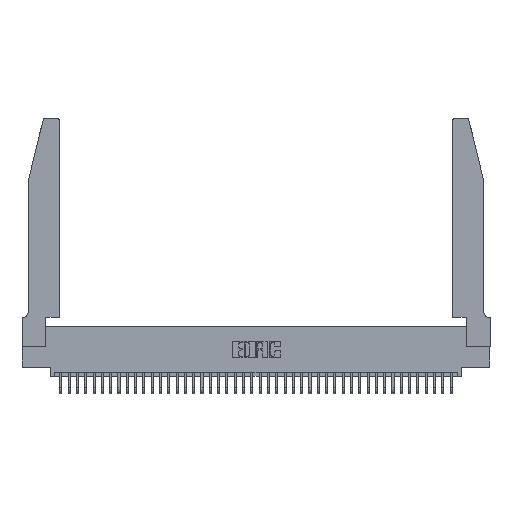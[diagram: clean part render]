
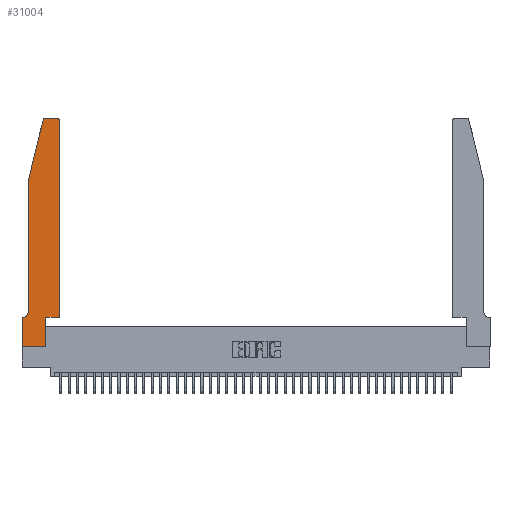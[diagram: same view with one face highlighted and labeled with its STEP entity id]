
A CAD part, top view. The second image highlights one B-rep face of the part: STEP entity #31004.
In plain terms, the highlighted planar face has unit normal (0, 0, 1).
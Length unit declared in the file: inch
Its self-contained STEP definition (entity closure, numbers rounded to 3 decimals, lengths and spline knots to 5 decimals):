
#137 = ORIENTED_EDGE ( 'NONE', *, *, #31049, .T. ) ;
#503 = ORIENTED_EDGE ( 'NONE', *, *, #36519, .T. ) ;
#614 = CARTESIAN_POINT ( 'NONE',  ( 0., 0., 0.37 ) ) ;
#627 = CARTESIAN_POINT ( 'NONE',  ( 0.2865, 0.35, 0.37 ) ) ;
#1128 = VERTEX_POINT ( 'NONE', #8726 ) ;
#1502 = LINE ( 'NONE', #24448, #2562 ) ;
#1801 = VERTEX_POINT ( 'NONE', #23933 ) ;
#1944 = VERTEX_POINT ( 'NONE', #18212 ) ;
#2562 = VECTOR ( 'NONE', #17711, 39.37008 ) ;
#2728 = DIRECTION ( 'NONE',  ( 0., 1., 0. ) ) ;
#3077 = ORIENTED_EDGE ( 'NONE', *, *, #26195, .T. ) ;
#4202 = ORIENTED_EDGE ( 'NONE', *, *, #9732, .T. ) ;
#4625 = VECTOR ( 'NONE', #2728, 39.37008 ) ;
#6936 = LINE ( 'NONE', #20820, #40426 ) ;
#8248 = CARTESIAN_POINT ( 'NONE',  ( 0.0755, 2., 0.37 ) ) ;
#8726 = CARTESIAN_POINT ( 'NONE',  ( 0., 0.35, 0.37 ) ) ;
#8835 = CARTESIAN_POINT ( 'NONE',  ( 0.284, 2.72, 0.37 ) ) ;
#8965 = CIRCLE ( 'NONE', #24056, 0.03 ) ;
#9063 = ORIENTED_EDGE ( 'NONE', *, *, #30540, .T. ) ;
#9194 = VERTEX_POINT ( 'NONE', #18408 ) ;
#9270 = EDGE_CURVE ( 'NONE', #25083, #10269, #41561, .T. ) ;
#9732 = EDGE_CURVE ( 'NONE', #1801, #9194, #25870, .T. ) ;
#10200 = EDGE_CURVE ( 'NONE', #9194, #11248, #6936, .T. ) ;
#10269 = VERTEX_POINT ( 'NONE', #11112 ) ;
#10352 = ORIENTED_EDGE ( 'NONE', *, *, #10200, .T. ) ;
#11086 = EDGE_CURVE ( 'NONE', #10269, #1801, #8965, .T. ) ;
#11112 = CARTESIAN_POINT ( 'NONE',  ( 0.284, 2.75, 0.37 ) ) ;
#11248 = VERTEX_POINT ( 'NONE', #39684 ) ;
#11329 = DIRECTION ( 'NONE',  ( 1., 0., 0. ) ) ;
#11650 = EDGE_CURVE ( 'NONE', #26159, #1128, #13074, .T. ) ;
#11720 = VECTOR ( 'NONE', #37430, 39.37008 ) ;
#12178 = DIRECTION ( 'NONE',  ( 1., 0., 0. ) ) ;
#12601 = CARTESIAN_POINT ( 'NONE',  ( 0., 0.35, 0.37 ) ) ;
#12748 = CARTESIAN_POINT ( 'NONE',  ( 0.2865, 0.35, 0.37 ) ) ;
#13074 = LINE ( 'NONE', #42562, #28809 ) ;
#13077 = CARTESIAN_POINT ( 'NONE',  ( 0.0055, 0.42, 0.37 ) ) ;
#13531 = LINE ( 'NONE', #12748, #4625 ) ;
#14582 = DIRECTION ( 'NONE',  ( 0., 0., 1. ) ) ;
#14614 = VECTOR ( 'NONE', #36022, 39.37008 ) ;
#14873 = VECTOR ( 'NONE', #35007, 39.37008 ) ;
#14917 = VECTOR ( 'NONE', #26003, 39.37008 ) ;
#14987 = CARTESIAN_POINT ( 'NONE',  ( 0.4205, 2.75, 0.37 ) ) ;
#15870 = CIRCLE ( 'NONE', #17442, 0.03 ) ;
#16011 = DIRECTION ( 'NONE',  ( 0., 0., 1. ) ) ;
#16172 = CIRCLE ( 'NONE', #18349, 0.07 ) ;
#16478 = DIRECTION ( 'NONE',  ( -1., 0., 0. ) ) ;
#16599 = LINE ( 'NONE', #31402, #24458 ) ;
#16724 = FACE_OUTER_BOUND ( 'NONE', #34205, .T. ) ;
#17442 = AXIS2_PLACEMENT_3D ( 'NONE', #34615, #14582, #37977 ) ;
#17683 = ORIENTED_EDGE ( 'NONE', *, *, #11086, .T. ) ;
#17711 = DIRECTION ( 'NONE',  ( 0., -1., 0. ) ) ;
#17792 = CARTESIAN_POINT ( 'NONE',  ( 0.2865, 0., 0.37 ) ) ;
#18212 = CARTESIAN_POINT ( 'NONE',  ( 0., 0., 0.37 ) ) ;
#18349 = AXIS2_PLACEMENT_3D ( 'NONE', #13077, #36478, #16478 ) ;
#18408 = CARTESIAN_POINT ( 'NONE',  ( 0.0755, 2., 0.37 ) ) ;
#19075 = DIRECTION ( 'NONE',  ( -1., 0., 0. ) ) ;
#19386 = CARTESIAN_POINT ( 'NONE',  ( 0.4505, 0.35, 0.37 ) ) ;
#20820 = CARTESIAN_POINT ( 'NONE',  ( 0.0755, 2., 0.37 ) ) ;
#21285 = ORIENTED_EDGE ( 'NONE', *, *, #28069, .T. ) ;
#21300 = VERTEX_POINT ( 'NONE', #42207 ) ;
#23660 = VERTEX_POINT ( 'NONE', #627 ) ;
#23933 = CARTESIAN_POINT ( 'NONE',  ( 0.25487, 2.72718, 0.37 ) ) ;
#24056 = AXIS2_PLACEMENT_3D ( 'NONE', #8835, #32252, #12178 ) ;
#24338 = CARTESIAN_POINT ( 'NONE',  ( 0.4505, 0.35, 0.37 ) ) ;
#24448 = CARTESIAN_POINT ( 'NONE',  ( 0., 0., 0.37 ) ) ;
#24458 = VECTOR ( 'NONE', #11329, 39.37008 ) ;
#25083 = VERTEX_POINT ( 'NONE', #14987 ) ;
#25870 = LINE ( 'NONE', #8248, #14873 ) ;
#26003 = DIRECTION ( 'NONE',  ( -1., 0., 0. ) ) ;
#26159 = VERTEX_POINT ( 'NONE', #34465 ) ;
#26195 = EDGE_CURVE ( 'NONE', #23660, #32619, #16599, .T. ) ;
#27463 = EDGE_CURVE ( 'NONE', #1944, #33893, #29569, .T. ) ;
#28069 = EDGE_CURVE ( 'NONE', #21300, #25083, #15870, .T. ) ;
#28809 = VECTOR ( 'NONE', #19075, 39.37008 ) ;
#29178 = ORIENTED_EDGE ( 'NONE', *, *, #9270, .T. ) ;
#29377 = CARTESIAN_POINT ( 'NONE',  ( 0.2605, 2.75, 0.37 ) ) ;
#29569 = LINE ( 'NONE', #614, #11720 ) ;
#30540 = EDGE_CURVE ( 'NONE', #11248, #26159, #16172, .T. ) ;
#31004 = ADVANCED_FACE ( 'NONE', ( #16724 ), #32521, .T. ) ;
#31011 = EDGE_CURVE ( 'NONE', #32619, #21300, #41275, .T. ) ;
#31049 = EDGE_CURVE ( 'NONE', #33893, #23660, #13531, .T. ) ;
#31402 = CARTESIAN_POINT ( 'NONE',  ( 0.4505, 0.35, 0.37 ) ) ;
#32252 = DIRECTION ( 'NONE',  ( 0., 0., 1. ) ) ;
#32521 = PLANE ( 'NONE',  #39886 ) ;
#32619 = VERTEX_POINT ( 'NONE', #24338 ) ;
#33494 = ORIENTED_EDGE ( 'NONE', *, *, #31011, .T. ) ;
#33893 = VERTEX_POINT ( 'NONE', #17792 ) ;
#34205 = EDGE_LOOP ( 'NONE', ( #29178, #17683, #4202, #10352, #9063, #38067, #503, #41913, #137, #3077, #33494, #21285 ) ) ;
#34249 = DIRECTION ( 'NONE',  ( 0., -1., 0. ) ) ;
#34465 = CARTESIAN_POINT ( 'NONE',  ( 0.0055, 0.35, 0.37 ) ) ;
#34615 = CARTESIAN_POINT ( 'NONE',  ( 0.4205, 2.72, 0.37 ) ) ;
#35007 = DIRECTION ( 'NONE',  ( -0.239, -0.971, 0. ) ) ;
#36022 = DIRECTION ( 'NONE',  ( 0., 1., 0. ) ) ;
#36478 = DIRECTION ( 'NONE',  ( 0., 0., -1. ) ) ;
#36519 = EDGE_CURVE ( 'NONE', #1128, #1944, #1502, .T. ) ;
#37430 = DIRECTION ( 'NONE',  ( 1., 0., 0. ) ) ;
#37977 = DIRECTION ( 'NONE',  ( 1., 0., 0. ) ) ;
#38067 = ORIENTED_EDGE ( 'NONE', *, *, #11650, .T. ) ;
#39382 = DIRECTION ( 'NONE',  ( 1., 0., 0. ) ) ;
#39684 = CARTESIAN_POINT ( 'NONE',  ( 0.0755, 0.42, 0.37 ) ) ;
#39886 = AXIS2_PLACEMENT_3D ( 'NONE', #12601, #16011, #39382 ) ;
#40426 = VECTOR ( 'NONE', #34249, 39.37008 ) ;
#41275 = LINE ( 'NONE', #19386, #14614 ) ;
#41561 = LINE ( 'NONE', #29377, #14917 ) ;
#41913 = ORIENTED_EDGE ( 'NONE', *, *, #27463, .T. ) ;
#42207 = CARTESIAN_POINT ( 'NONE',  ( 0.4505, 2.72, 0.37 ) ) ;
#42562 = CARTESIAN_POINT ( 'NONE',  ( 0.0755, 0.35, 0.37 ) ) ;
